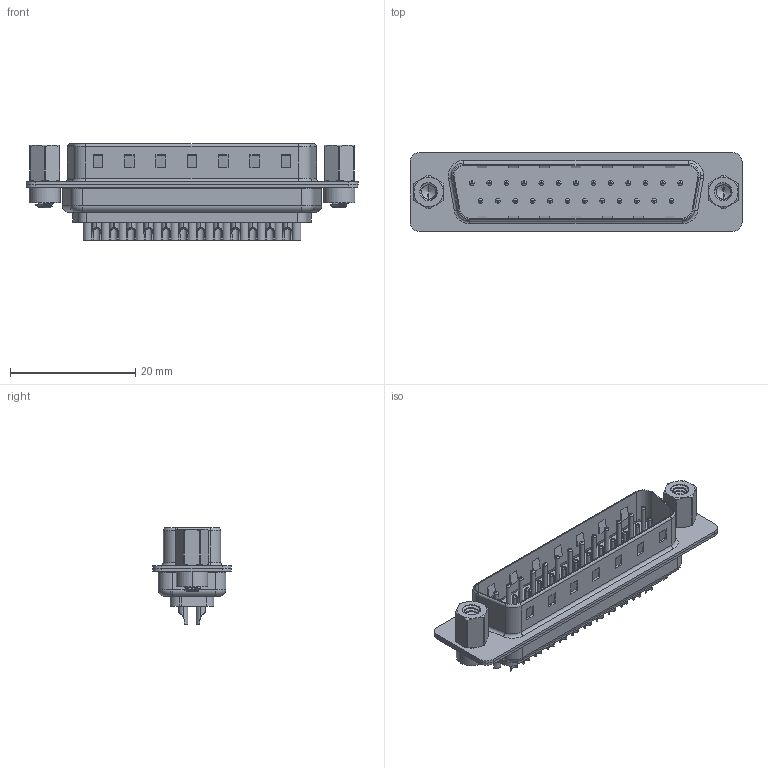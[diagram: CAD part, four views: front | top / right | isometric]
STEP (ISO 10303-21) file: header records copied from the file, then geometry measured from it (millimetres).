
FILE_DESCRIPTION (( 'STEP AP203' ), '1' );
FILE_NAME ('627-025-322-063.STEP', '2020-07-14T20:10:37', ( '' ), ( '' ), 'SwSTEP 2.0', 'SolidWorks 2020', '' );
FILE_SCHEMA (( 'CONFIG_CONTROL_DESIGN' ));
Length unit declared in the file: millimetre
Products named in the file (8): 627-025-322-063; 627 Shell Rear_25 Contacts; 627 Contact Row 2_22L; 627 Contact Row 1_22L; 627 4-40 Threaded Rivet; 627 Shell Front_25 Contacts; 627 4-40 Hex Standoff; 627 Housing_25 LP
Assembly tree (32 placements, depth 2):
  627-025-322-063
    627 Housing_25 LP
    627 Shell Front_25 Contacts
    627 Shell Rear_25 Contacts
    627 Contact Row 1_22L  x13
    627 Contact Row 2_22L  x12
    627 4-40 Threaded Rivet  x2
    627 4-40 Hex Standoff  x2
Bounding box: 53 x 12.6 x 15.35 mm (x, y, z)
Volume: 2898.3 mm3; surface area: 8328.2 mm2
Topology: 32 solids, 32 shells, 2098 faces, 5395 edges, 3422 vertices
Faces by surface type: cylinder 932, torus 575, plane 543, cone 30, bspline 18
Entity records: 27345 total; most frequent: CARTESIAN_POINT 8172, DIRECTION 3895, ORIENTED_EDGE 3570, EDGE_CURVE 1785, AXIS2_PLACEMENT_3D 1528, VERTEX_POINT 1144, EDGE_LOOP 869, VECTOR 839
